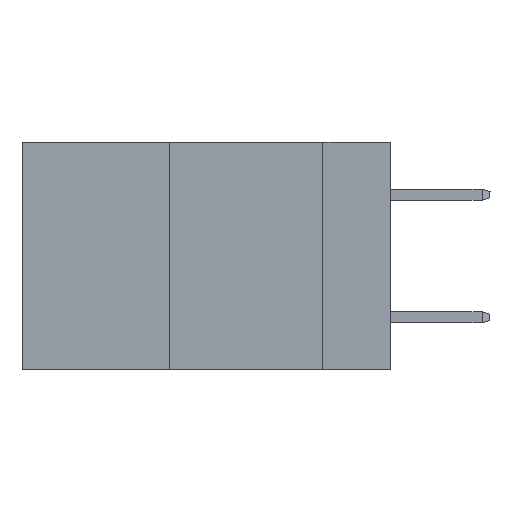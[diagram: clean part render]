
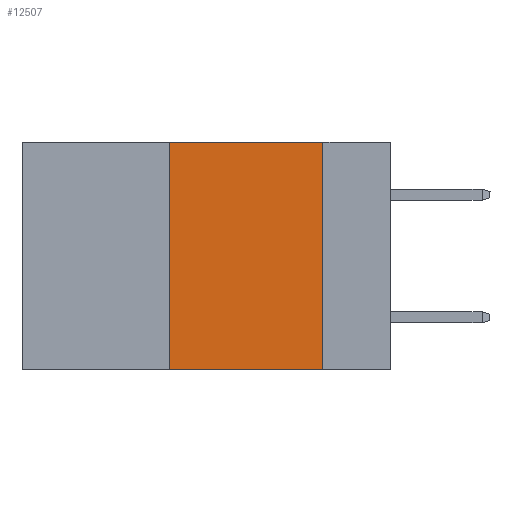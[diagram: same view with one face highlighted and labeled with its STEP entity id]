
A CAD part, left-side view. The second image highlights one B-rep face of the part: STEP entity #12507.
In plain terms, the highlighted planar face has unit normal (-1, 0, 0).
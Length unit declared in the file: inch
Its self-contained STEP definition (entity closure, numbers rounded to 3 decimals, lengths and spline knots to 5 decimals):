
#468 = ORIENTED_EDGE ( 'NONE', *, *, #4218, .F. ) ;
#596 = PLANE ( 'NONE',  #5512 ) ;
#889 = LINE ( 'NONE', #10637, #16973 ) ;
#1466 = CARTESIAN_POINT ( 'NONE',  ( 0., 0.36, -0.37 ) ) ;
#1515 = DIRECTION ( 'NONE',  ( 0., 0., -1. ) ) ;
#1608 = CARTESIAN_POINT ( 'NONE',  ( 0., 0.6, -0.37 ) ) ;
#1842 = VECTOR ( 'NONE', #1515, 39.37008 ) ;
#2188 = CARTESIAN_POINT ( 'NONE',  ( 0., 0.6, 0. ) ) ;
#2311 = ORIENTED_EDGE ( 'NONE', *, *, #5763, .F. ) ;
#3510 = LINE ( 'NONE', #1608, #7123 ) ;
#4076 = VECTOR ( 'NONE', #5494, 39.37008 ) ;
#4218 = EDGE_CURVE ( 'NONE', #8857, #18747, #889, .T. ) ;
#4375 = VERTEX_POINT ( 'NONE', #4646 ) ;
#4645 = ORIENTED_EDGE ( 'NONE', *, *, #7235, .T. ) ;
#4646 = CARTESIAN_POINT ( 'NONE',  ( 0., 0.11, -0.37 ) ) ;
#5494 = DIRECTION ( 'NONE',  ( 0., 0., 1. ) ) ;
#5512 = AXIS2_PLACEMENT_3D ( 'NONE', #2188, #16016, #9762 ) ;
#5763 = EDGE_CURVE ( 'NONE', #15539, #8857, #16015, .T. ) ;
#6034 = ORIENTED_EDGE ( 'NONE', *, *, #6424, .F. ) ;
#6424 = EDGE_CURVE ( 'NONE', #18747, #4375, #14265, .T. ) ;
#7123 = VECTOR ( 'NONE', #12459, 39.37008 ) ;
#7235 = EDGE_CURVE ( 'NONE', #15539, #4375, #3510, .T. ) ;
#7455 = CARTESIAN_POINT ( 'NONE',  ( 0., 0.36, 0. ) ) ;
#8857 = VERTEX_POINT ( 'NONE', #7455 ) ;
#9762 = DIRECTION ( 'NONE',  ( 0., 0., -1. ) ) ;
#10637 = CARTESIAN_POINT ( 'NONE',  ( 0., 0.6, 0. ) ) ;
#11501 = EDGE_LOOP ( 'NONE', ( #6034, #468, #2311, #4645 ) ) ;
#12459 = DIRECTION ( 'NONE',  ( 0., -1., 0. ) ) ;
#12507 = ADVANCED_FACE ( 'NONE', ( #17543 ), #596, .F. ) ;
#13261 = CARTESIAN_POINT ( 'NONE',  ( 0., 0.36, 0. ) ) ;
#14265 = LINE ( 'NONE', #15547, #1842 ) ;
#15539 = VERTEX_POINT ( 'NONE', #1466 ) ;
#15547 = CARTESIAN_POINT ( 'NONE',  ( 0., 0.11, 0. ) ) ;
#16015 = LINE ( 'NONE', #13261, #4076 ) ;
#16016 = DIRECTION ( 'NONE',  ( 1., 0., 0. ) ) ;
#16973 = VECTOR ( 'NONE', #18233, 39.37008 ) ;
#17543 = FACE_OUTER_BOUND ( 'NONE', #11501, .T. ) ;
#18233 = DIRECTION ( 'NONE',  ( 0., -1., 0. ) ) ;
#18747 = VERTEX_POINT ( 'NONE', #19657 ) ;
#19657 = CARTESIAN_POINT ( 'NONE',  ( 0., 0.11, 0. ) ) ;
